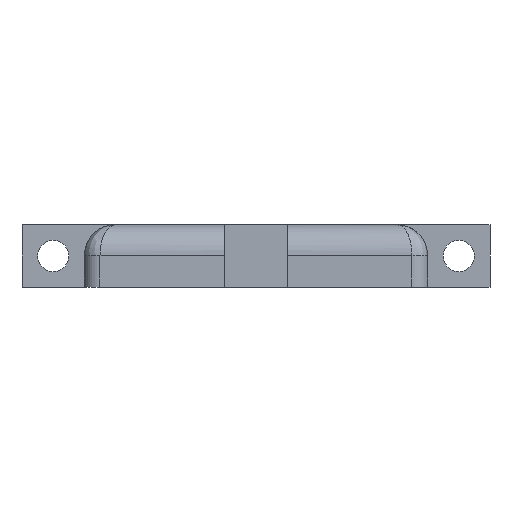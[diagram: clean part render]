
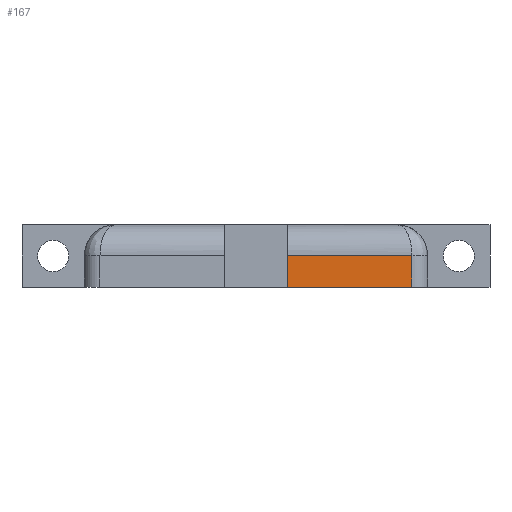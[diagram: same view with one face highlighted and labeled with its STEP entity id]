
A CAD part, left-side view. The second image highlights one B-rep face of the part: STEP entity #167.
In plain terms, the highlighted planar face has unit normal (-1, 0, 0).
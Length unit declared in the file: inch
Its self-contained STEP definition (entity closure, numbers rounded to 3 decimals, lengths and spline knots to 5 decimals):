
#84 = CARTESIAN_POINT ( 'NONE',  ( 0., -1.3, 0. ) ) ;
#167 = ADVANCED_FACE ( 'NONE', ( #1386 ), #1357, .F. ) ;
#199 = DIRECTION ( 'NONE',  ( 1., 0., 0. ) ) ;
#207 = EDGE_CURVE ( 'NONE', #424, #283, #647, .T. ) ;
#267 = LINE ( 'NONE', #84, #1587 ) ;
#283 = VERTEX_POINT ( 'NONE', #1457 ) ;
#358 = CARTESIAN_POINT ( 'NONE',  ( 0., -1.3, 0. ) ) ;
#371 = CARTESIAN_POINT ( 'NONE',  ( 0., -1.3, 0.20315 ) ) ;
#396 = VERTEX_POINT ( 'NONE', #371 ) ;
#424 = VERTEX_POINT ( 'NONE', #358 ) ;
#448 = DIRECTION ( 'NONE',  ( 0., 0., 1. ) ) ;
#562 = VECTOR ( 'NONE', #448, 39.37008 ) ;
#616 = DIRECTION ( 'NONE',  ( 0., 0., 1. ) ) ;
#647 = LINE ( 'NONE', #1221, #1547 ) ;
#649 = EDGE_LOOP ( 'NONE', ( #1620, #1395, #1230, #1417 ) ) ;
#702 = DIRECTION ( 'NONE',  ( 0., 1., 0. ) ) ;
#757 = VECTOR ( 'NONE', #1034, 39.37008 ) ;
#815 = EDGE_CURVE ( 'NONE', #424, #396, #267, .T. ) ;
#927 = CARTESIAN_POINT ( 'NONE',  ( 0., -1.3, 0.20315 ) ) ;
#940 = LINE ( 'NONE', #1220, #562 ) ;
#1034 = DIRECTION ( 'NONE',  ( 0., 1., 0. ) ) ;
#1105 = CARTESIAN_POINT ( 'NONE',  ( 0., 0., 0.4 ) ) ;
#1216 = VERTEX_POINT ( 'NONE', #1422 ) ;
#1220 = CARTESIAN_POINT ( 'NONE',  ( 0., -2.1, 0.4 ) ) ;
#1221 = CARTESIAN_POINT ( 'NONE',  ( 0., 0., 0. ) ) ;
#1230 = ORIENTED_EDGE ( 'NONE', *, *, #1310, .T. ) ;
#1303 = AXIS2_PLACEMENT_3D ( 'NONE', #1105, #199, #702 ) ;
#1310 = EDGE_CURVE ( 'NONE', #1216, #396, #1598, .T. ) ;
#1357 = PLANE ( 'NONE',  #1303 ) ;
#1386 = FACE_OUTER_BOUND ( 'NONE', #649, .T. ) ;
#1395 = ORIENTED_EDGE ( 'NONE', *, *, #1638, .T. ) ;
#1417 = ORIENTED_EDGE ( 'NONE', *, *, #815, .F. ) ;
#1422 = CARTESIAN_POINT ( 'NONE',  ( 0., -2.1, 0.20315 ) ) ;
#1457 = CARTESIAN_POINT ( 'NONE',  ( 0., -2.1, 0. ) ) ;
#1465 = DIRECTION ( 'NONE',  ( 0., -1., 0. ) ) ;
#1547 = VECTOR ( 'NONE', #1465, 39.37008 ) ;
#1587 = VECTOR ( 'NONE', #616, 39.37008 ) ;
#1598 = LINE ( 'NONE', #927, #757 ) ;
#1620 = ORIENTED_EDGE ( 'NONE', *, *, #207, .T. ) ;
#1638 = EDGE_CURVE ( 'NONE', #283, #1216, #940, .T. ) ;
